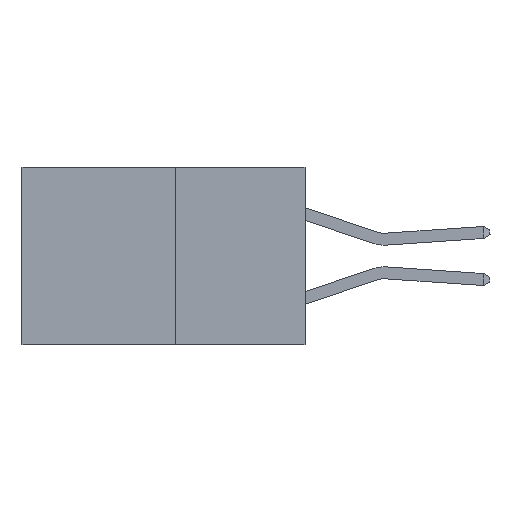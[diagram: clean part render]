
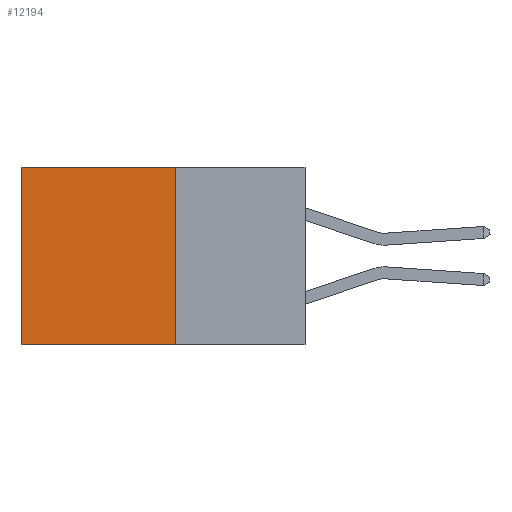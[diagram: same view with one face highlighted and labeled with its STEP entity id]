
A CAD part, left-side view. The second image highlights one B-rep face of the part: STEP entity #12194.
In plain terms, the highlighted planar face has unit normal (-1, 0, 0).
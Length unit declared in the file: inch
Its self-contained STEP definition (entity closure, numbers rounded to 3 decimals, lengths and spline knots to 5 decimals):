
#376 = DIRECTION ( 'NONE',  ( 0., 0., -1. ) ) ;
#1190 = ORIENTED_EDGE ( 'NONE', *, *, #19595, .T. ) ;
#2094 = VECTOR ( 'NONE', #15841, 39.37008 ) ;
#2455 = DIRECTION ( 'NONE',  ( 0., 0., -1. ) ) ;
#2892 = CARTESIAN_POINT ( 'NONE',  ( 0.277, 0.27, -0.37 ) ) ;
#3171 = EDGE_LOOP ( 'NONE', ( #1190, #18591, #15018, #25638 ) ) ;
#3655 = CARTESIAN_POINT ( 'NONE',  ( 0.277, 0.27, -0.37 ) ) ;
#4699 = EDGE_CURVE ( 'NONE', #15915, #20061, #8928, .T. ) ;
#5880 = EDGE_CURVE ( 'NONE', #15915, #25655, #9190, .T. ) ;
#8536 = VECTOR ( 'NONE', #2455, 39.37008 ) ;
#8667 = PLANE ( 'NONE',  #17123 ) ;
#8928 = LINE ( 'NONE', #24259, #19204 ) ;
#9190 = LINE ( 'NONE', #2892, #8536 ) ;
#10698 = VERTEX_POINT ( 'NONE', #24707 ) ;
#11012 = CARTESIAN_POINT ( 'NONE',  ( 0.277, 0.59, 0. ) ) ;
#12194 = ADVANCED_FACE ( 'NONE', ( #20185 ), #8667, .F. ) ;
#12745 = DIRECTION ( 'NONE',  ( 1., 0., 0. ) ) ;
#13100 = LINE ( 'NONE', #25924, #2094 ) ;
#14083 = CARTESIAN_POINT ( 'NONE',  ( 0.277, 0.27, -0.37 ) ) ;
#15018 = ORIENTED_EDGE ( 'NONE', *, *, #5880, .F. ) ;
#15841 = DIRECTION ( 'NONE',  ( 0., 0., -1. ) ) ;
#15915 = VERTEX_POINT ( 'NONE', #22662 ) ;
#16128 = DIRECTION ( 'NONE',  ( 0., 1., 0. ) ) ;
#17123 = AXIS2_PLACEMENT_3D ( 'NONE', #24893, #12745, #376 ) ;
#18591 = ORIENTED_EDGE ( 'NONE', *, *, #23966, .F. ) ;
#19204 = VECTOR ( 'NONE', #24241, 39.37008 ) ;
#19595 = EDGE_CURVE ( 'NONE', #20061, #10698, #13100, .T. ) ;
#20061 = VERTEX_POINT ( 'NONE', #11012 ) ;
#20185 = FACE_OUTER_BOUND ( 'NONE', #3171, .T. ) ;
#22662 = CARTESIAN_POINT ( 'NONE',  ( 0.277, 0.27, 0. ) ) ;
#23966 = EDGE_CURVE ( 'NONE', #25655, #10698, #25475, .T. ) ;
#24241 = DIRECTION ( 'NONE',  ( 0., 1., 0. ) ) ;
#24259 = CARTESIAN_POINT ( 'NONE',  ( 0.277, 0.27, 0. ) ) ;
#24707 = CARTESIAN_POINT ( 'NONE',  ( 0.277, 0.59, -0.37 ) ) ;
#24821 = VECTOR ( 'NONE', #16128, 39.37008 ) ;
#24893 = CARTESIAN_POINT ( 'NONE',  ( 0.277, 0.27, -0.37 ) ) ;
#25475 = LINE ( 'NONE', #14083, #24821 ) ;
#25638 = ORIENTED_EDGE ( 'NONE', *, *, #4699, .T. ) ;
#25655 = VERTEX_POINT ( 'NONE', #3655 ) ;
#25924 = CARTESIAN_POINT ( 'NONE',  ( 0.277, 0.59, -0.37 ) ) ;
